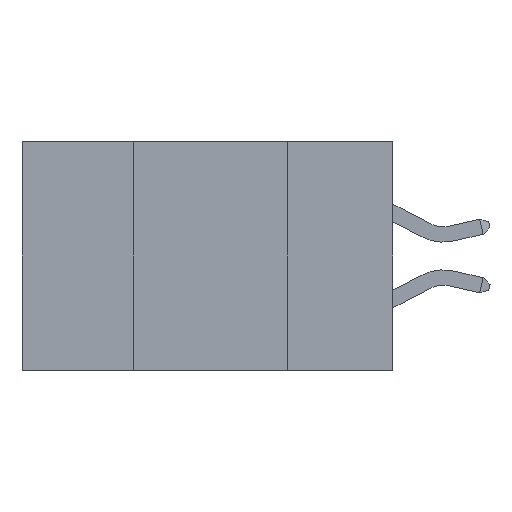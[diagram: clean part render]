
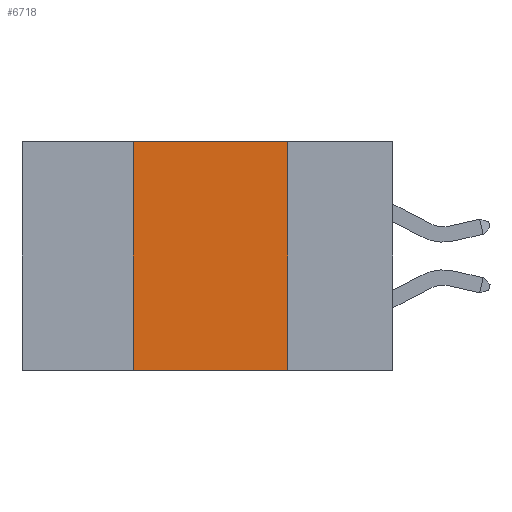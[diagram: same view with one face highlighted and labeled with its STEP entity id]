
A CAD part, left-side view. The second image highlights one B-rep face of the part: STEP entity #6718.
In plain terms, the highlighted planar face has unit normal (-1, 0, 0).
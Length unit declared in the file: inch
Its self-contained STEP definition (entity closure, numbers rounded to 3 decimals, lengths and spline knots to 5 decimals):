
#59 = VERTEX_POINT ( 'NONE', #2234 ) ;
#398 = CARTESIAN_POINT ( 'NONE',  ( 0., 0.42, 0. ) ) ;
#420 = DIRECTION ( 'NONE',  ( 0., -1., 0. ) ) ;
#753 = DIRECTION ( 'NONE',  ( 0., -1., 0. ) ) ;
#776 = ORIENTED_EDGE ( 'NONE', *, *, #9954, .T. ) ;
#1404 = CARTESIAN_POINT ( 'NONE',  ( 0., 0.17, 0. ) ) ;
#1918 = VERTEX_POINT ( 'NONE', #1404 ) ;
#1997 = LINE ( 'NONE', #2078, #10389 ) ;
#2078 = CARTESIAN_POINT ( 'NONE',  ( 0., 0.42, 0. ) ) ;
#2234 = CARTESIAN_POINT ( 'NONE',  ( 0., 0.17, -0.37 ) ) ;
#2505 = EDGE_CURVE ( 'NONE', #1918, #59, #5034, .T. ) ;
#2609 = VECTOR ( 'NONE', #6648, 39.37008 ) ;
#2715 = CARTESIAN_POINT ( 'NONE',  ( 0., 0.6, 0. ) ) ;
#2738 = ORIENTED_EDGE ( 'NONE', *, *, #9231, .F. ) ;
#3130 = CARTESIAN_POINT ( 'NONE',  ( 0., 0.6, -0.37 ) ) ;
#3624 = DIRECTION ( 'NONE',  ( 1., 0., 0. ) ) ;
#4020 = ORIENTED_EDGE ( 'NONE', *, *, #2505, .F. ) ;
#4350 = CARTESIAN_POINT ( 'NONE',  ( 0., 0.6, 0. ) ) ;
#4452 = EDGE_CURVE ( 'NONE', #8629, #8952, #1997, .T. ) ;
#4485 = LINE ( 'NONE', #4350, #10938 ) ;
#5034 = LINE ( 'NONE', #7511, #2609 ) ;
#5410 = DIRECTION ( 'NONE',  ( 0., 0., -1. ) ) ;
#6255 = ORIENTED_EDGE ( 'NONE', *, *, #4452, .F. ) ;
#6648 = DIRECTION ( 'NONE',  ( 0., 0., -1. ) ) ;
#6696 = FACE_OUTER_BOUND ( 'NONE', #6812, .T. ) ;
#6718 = ADVANCED_FACE ( 'NONE', ( #6696 ), #8052, .F. ) ;
#6812 = EDGE_LOOP ( 'NONE', ( #4020, #2738, #6255, #776 ) ) ;
#6896 = CARTESIAN_POINT ( 'NONE',  ( 0., 0.42, -0.37 ) ) ;
#6924 = VECTOR ( 'NONE', #420, 39.37008 ) ;
#7511 = CARTESIAN_POINT ( 'NONE',  ( 0., 0.17, 0. ) ) ;
#8052 = PLANE ( 'NONE',  #8132 ) ;
#8129 = LINE ( 'NONE', #3130, #6924 ) ;
#8132 = AXIS2_PLACEMENT_3D ( 'NONE', #2715, #3624, #5410 ) ;
#8629 = VERTEX_POINT ( 'NONE', #6896 ) ;
#8952 = VERTEX_POINT ( 'NONE', #398 ) ;
#9231 = EDGE_CURVE ( 'NONE', #8952, #1918, #4485, .T. ) ;
#9817 = DIRECTION ( 'NONE',  ( 0., 0., 1. ) ) ;
#9954 = EDGE_CURVE ( 'NONE', #8629, #59, #8129, .T. ) ;
#10389 = VECTOR ( 'NONE', #9817, 39.37008 ) ;
#10938 = VECTOR ( 'NONE', #753, 39.37008 ) ;
